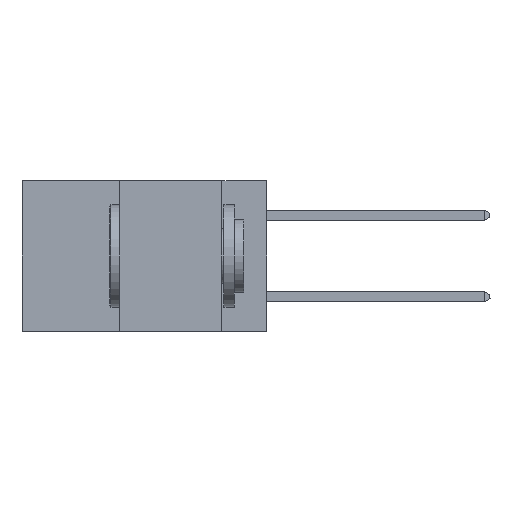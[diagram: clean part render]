
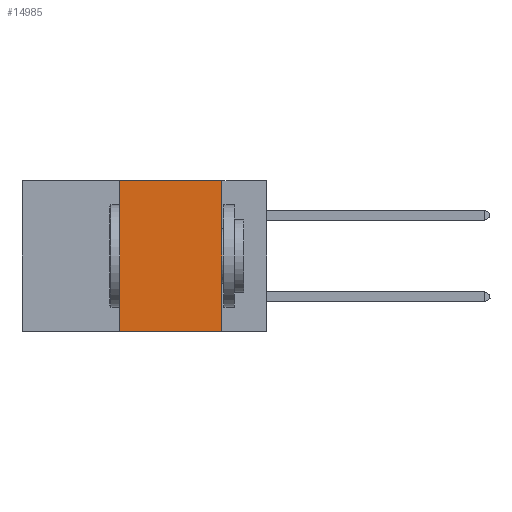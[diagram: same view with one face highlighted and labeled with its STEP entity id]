
A CAD part, left-side view. The second image highlights one B-rep face of the part: STEP entity #14985.
In plain terms, the highlighted planar face has unit normal (-1, 0, 0).
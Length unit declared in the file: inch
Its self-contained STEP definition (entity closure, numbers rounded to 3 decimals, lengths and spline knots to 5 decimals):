
#51 = DIRECTION ( 'NONE',  ( 0., 0., 1. ) ) ;
#747 = VECTOR ( 'NONE', #20996, 39.37008 ) ;
#3043 = VECTOR ( 'NONE', #24297, 39.37008 ) ;
#3842 = CARTESIAN_POINT ( 'NONE',  ( 0., 0.6, -0.37 ) ) ;
#5478 = LINE ( 'NONE', #3842, #3043 ) ;
#5499 = DIRECTION ( 'NONE',  ( 0., 0., -1. ) ) ;
#5870 = ORIENTED_EDGE ( 'NONE', *, *, #28156, .F. ) ;
#6718 = CARTESIAN_POINT ( 'NONE',  ( 0., 0.36, 0. ) ) ;
#8099 = VERTEX_POINT ( 'NONE', #32479 ) ;
#8161 = CARTESIAN_POINT ( 'NONE',  ( 0., 0.36, 0. ) ) ;
#8829 = ORIENTED_EDGE ( 'NONE', *, *, #14996, .F. ) ;
#9832 = VERTEX_POINT ( 'NONE', #28736 ) ;
#10186 = VERTEX_POINT ( 'NONE', #6718 ) ;
#12960 = CARTESIAN_POINT ( 'NONE',  ( 0., 0.6, 0. ) ) ;
#13176 = CARTESIAN_POINT ( 'NONE',  ( 0., 0.11, 0. ) ) ;
#14271 = CARTESIAN_POINT ( 'NONE',  ( 0., 0.6, 0. ) ) ;
#14703 = DIRECTION ( 'NONE',  ( 0., -1., 0. ) ) ;
#14838 = AXIS2_PLACEMENT_3D ( 'NONE', #12960, #30820, #5499 ) ;
#14905 = VECTOR ( 'NONE', #14703, 39.37008 ) ;
#14985 = ADVANCED_FACE ( 'NONE', ( #21450 ), #28271, .F. ) ;
#14996 = EDGE_CURVE ( 'NONE', #9832, #10186, #20249, .T. ) ;
#15325 = EDGE_CURVE ( 'NONE', #9832, #8099, #5478, .T. ) ;
#18743 = VERTEX_POINT ( 'NONE', #29235 ) ;
#20249 = LINE ( 'NONE', #8161, #29831 ) ;
#20370 = LINE ( 'NONE', #13176, #747 ) ;
#20996 = DIRECTION ( 'NONE',  ( 0., 0., -1. ) ) ;
#21450 = FACE_OUTER_BOUND ( 'NONE', #24289, .T. ) ;
#22133 = ORIENTED_EDGE ( 'NONE', *, *, #15325, .T. ) ;
#22503 = LINE ( 'NONE', #14271, #14905 ) ;
#23521 = ORIENTED_EDGE ( 'NONE', *, *, #24696, .F. ) ;
#24289 = EDGE_LOOP ( 'NONE', ( #23521, #5870, #8829, #22133 ) ) ;
#24297 = DIRECTION ( 'NONE',  ( 0., -1., 0. ) ) ;
#24696 = EDGE_CURVE ( 'NONE', #18743, #8099, #20370, .T. ) ;
#28156 = EDGE_CURVE ( 'NONE', #10186, #18743, #22503, .T. ) ;
#28271 = PLANE ( 'NONE',  #14838 ) ;
#28736 = CARTESIAN_POINT ( 'NONE',  ( 0., 0.36, -0.37 ) ) ;
#29235 = CARTESIAN_POINT ( 'NONE',  ( 0., 0.11, 0. ) ) ;
#29831 = VECTOR ( 'NONE', #51, 39.37008 ) ;
#30820 = DIRECTION ( 'NONE',  ( 1., 0., 0. ) ) ;
#32479 = CARTESIAN_POINT ( 'NONE',  ( 0., 0.11, -0.37 ) ) ;
